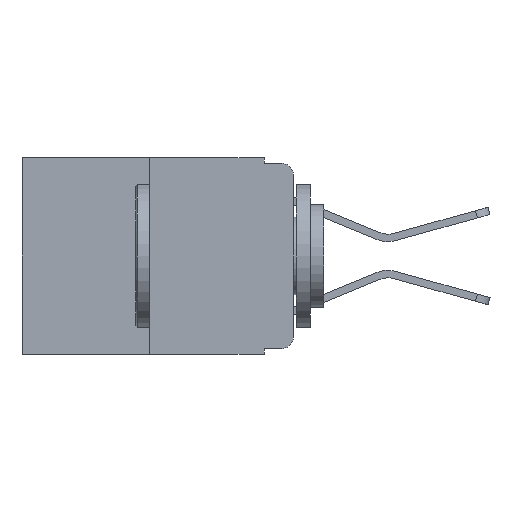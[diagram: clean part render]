
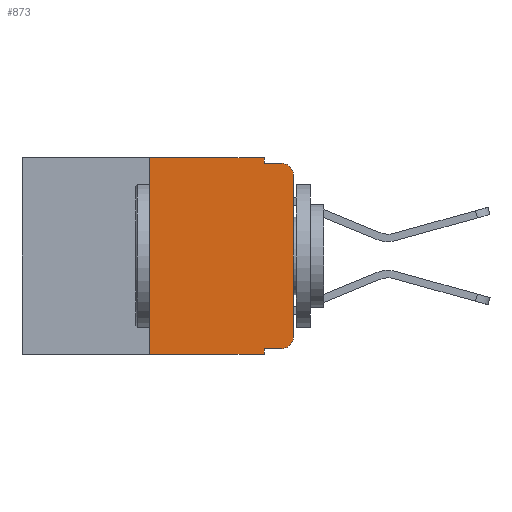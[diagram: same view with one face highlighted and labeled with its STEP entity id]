
A CAD part, left-side view. The second image highlights one B-rep face of the part: STEP entity #873.
In plain terms, the highlighted planar face has unit normal (-1, 0, 0).
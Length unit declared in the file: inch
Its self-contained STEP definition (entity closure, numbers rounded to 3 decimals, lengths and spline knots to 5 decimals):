
#127 = AXIS2_PLACEMENT_3D ( 'NONE', #13222, #1479, #10165 ) ;
#327 = VERTEX_POINT ( 'NONE', #7796 ) ;
#355 = CARTESIAN_POINT ( 'NONE',  ( 0., 0.25, -0.343 ) ) ;
#873 = ADVANCED_FACE ( 'NONE', ( #3272 ), #4515, .F. ) ;
#983 = DIRECTION ( 'NONE',  ( 0., 0., -1. ) ) ;
#1389 = ORIENTED_EDGE ( 'NONE', *, *, #9696, .T. ) ;
#1479 = DIRECTION ( 'NONE',  ( 1., 0., 0. ) ) ;
#1544 = CARTESIAN_POINT ( 'NONE',  ( 0., 0.051, -0.333 ) ) ;
#2011 = VERTEX_POINT ( 'NONE', #1544 ) ;
#2020 = CARTESIAN_POINT ( 'NONE',  ( 0., 0.02, -0.313 ) ) ;
#2175 = ORIENTED_EDGE ( 'NONE', *, *, #8054, .T. ) ;
#2196 = LINE ( 'NONE', #10213, #13044 ) ;
#2372 = AXIS2_PLACEMENT_3D ( 'NONE', #2020, #11763, #5278 ) ;
#2453 = CARTESIAN_POINT ( 'NONE',  ( 0., 0., 0. ) ) ;
#2547 = CARTESIAN_POINT ( 'NONE',  ( 0., 0.473, -0.343 ) ) ;
#2862 = VERTEX_POINT ( 'NONE', #6341 ) ;
#3072 = CIRCLE ( 'NONE', #5568, 0.02 ) ;
#3186 = DIRECTION ( 'NONE',  ( 0., 0., -1. ) ) ;
#3223 = LINE ( 'NONE', #8744, #9686 ) ;
#3272 = FACE_OUTER_BOUND ( 'NONE', #5026, .T. ) ;
#3273 = CARTESIAN_POINT ( 'NONE',  ( 0., 0.051, 0. ) ) ;
#3655 = ORIENTED_EDGE ( 'NONE', *, *, #5386, .F. ) ;
#4094 = VECTOR ( 'NONE', #5920, 39.37008 ) ;
#4178 = EDGE_CURVE ( 'NONE', #2011, #7075, #10985, .T. ) ;
#4372 = LINE ( 'NONE', #7074, #11822 ) ;
#4390 = VERTEX_POINT ( 'NONE', #12680 ) ;
#4432 = VECTOR ( 'NONE', #9004, 39.37008 ) ;
#4478 = LINE ( 'NONE', #5046, #12107 ) ;
#4515 = PLANE ( 'NONE',  #127 ) ;
#4577 = DIRECTION ( 'NONE',  ( 0., 0., 1. ) ) ;
#4743 = VERTEX_POINT ( 'NONE', #12072 ) ;
#4761 = LINE ( 'NONE', #2547, #4432 ) ;
#4918 = ORIENTED_EDGE ( 'NONE', *, *, #12527, .F. ) ;
#5000 = CARTESIAN_POINT ( 'NONE',  ( 0., 0.051, 0. ) ) ;
#5026 = EDGE_LOOP ( 'NONE', ( #6454, #10559, #4918, #8182, #8023, #3655, #1389, #7250, #2175, #13964 ) ) ;
#5046 = CARTESIAN_POINT ( 'NONE',  ( 0., 0.051, -0.333 ) ) ;
#5278 = DIRECTION ( 'NONE',  ( 0., 0., -1. ) ) ;
#5331 = VECTOR ( 'NONE', #4577, 39.37008 ) ;
#5386 = EDGE_CURVE ( 'NONE', #10908, #10377, #4372, .T. ) ;
#5417 = DIRECTION ( 'NONE',  ( 0., -1., 0. ) ) ;
#5568 = AXIS2_PLACEMENT_3D ( 'NONE', #8751, #9810, #983 ) ;
#5920 = DIRECTION ( 'NONE',  ( 0., 0., -1. ) ) ;
#6341 = CARTESIAN_POINT ( 'NONE',  ( 0., 0.051, 0. ) ) ;
#6454 = ORIENTED_EDGE ( 'NONE', *, *, #7702, .T. ) ;
#6464 = CARTESIAN_POINT ( 'NONE',  ( 0., 0.051, -0.01 ) ) ;
#6715 = LINE ( 'NONE', #2453, #5331 ) ;
#6854 = CIRCLE ( 'NONE', #2372, 0.02 ) ;
#7074 = CARTESIAN_POINT ( 'NONE',  ( 0., 0.25, 0. ) ) ;
#7075 = VERTEX_POINT ( 'NONE', #11156 ) ;
#7114 = DIRECTION ( 'NONE',  ( 0., 0., 1. ) ) ;
#7250 = ORIENTED_EDGE ( 'NONE', *, *, #4178, .F. ) ;
#7336 = VERTEX_POINT ( 'NONE', #6464 ) ;
#7702 = EDGE_CURVE ( 'NONE', #4390, #9623, #6715, .T. ) ;
#7796 = CARTESIAN_POINT ( 'NONE',  ( 0., 0.02, -0.01 ) ) ;
#8023 = ORIENTED_EDGE ( 'NONE', *, *, #12784, .F. ) ;
#8054 = EDGE_CURVE ( 'NONE', #2011, #4743, #4478, .T. ) ;
#8182 = ORIENTED_EDGE ( 'NONE', *, *, #9835, .F. ) ;
#8235 = EDGE_CURVE ( 'NONE', #4743, #4390, #6854, .T. ) ;
#8744 = CARTESIAN_POINT ( 'NONE',  ( 0., 0.051, -0.01 ) ) ;
#8751 = CARTESIAN_POINT ( 'NONE',  ( 0., 0.02, -0.03 ) ) ;
#9004 = DIRECTION ( 'NONE',  ( 0., -1., 0. ) ) ;
#9281 = DIRECTION ( 'NONE',  ( 0., -1., 0. ) ) ;
#9623 = VERTEX_POINT ( 'NONE', #11071 ) ;
#9686 = VECTOR ( 'NONE', #5417, 39.37008 ) ;
#9696 = EDGE_CURVE ( 'NONE', #10908, #7075, #4761, .T. ) ;
#9810 = DIRECTION ( 'NONE',  ( -1., 0., 0. ) ) ;
#9834 = VECTOR ( 'NONE', #3186, 39.37008 ) ;
#9835 = EDGE_CURVE ( 'NONE', #2862, #7336, #10207, .T. ) ;
#9985 = EDGE_CURVE ( 'NONE', #9623, #327, #3072, .T. ) ;
#10165 = DIRECTION ( 'NONE',  ( 0., 0., -1. ) ) ;
#10207 = LINE ( 'NONE', #5000, #4094 ) ;
#10213 = CARTESIAN_POINT ( 'NONE',  ( 0., 0.473, 0. ) ) ;
#10266 = CARTESIAN_POINT ( 'NONE',  ( 0., 0.25, 0. ) ) ;
#10377 = VERTEX_POINT ( 'NONE', #10266 ) ;
#10559 = ORIENTED_EDGE ( 'NONE', *, *, #9985, .T. ) ;
#10908 = VERTEX_POINT ( 'NONE', #355 ) ;
#10985 = LINE ( 'NONE', #3273, #9834 ) ;
#11071 = CARTESIAN_POINT ( 'NONE',  ( 0., 0., -0.03 ) ) ;
#11156 = CARTESIAN_POINT ( 'NONE',  ( 0., 0.051, -0.343 ) ) ;
#11407 = DIRECTION ( 'NONE',  ( 0., -1., 0. ) ) ;
#11763 = DIRECTION ( 'NONE',  ( -1., 0., 0. ) ) ;
#11822 = VECTOR ( 'NONE', #7114, 39.37008 ) ;
#12072 = CARTESIAN_POINT ( 'NONE',  ( 0., 0.02, -0.333 ) ) ;
#12107 = VECTOR ( 'NONE', #9281, 39.37008 ) ;
#12527 = EDGE_CURVE ( 'NONE', #7336, #327, #3223, .T. ) ;
#12680 = CARTESIAN_POINT ( 'NONE',  ( 0., 0., -0.313 ) ) ;
#12784 = EDGE_CURVE ( 'NONE', #10377, #2862, #2196, .T. ) ;
#13044 = VECTOR ( 'NONE', #11407, 39.37008 ) ;
#13222 = CARTESIAN_POINT ( 'NONE',  ( 0., 0.473, 0. ) ) ;
#13964 = ORIENTED_EDGE ( 'NONE', *, *, #8235, .T. ) ;
